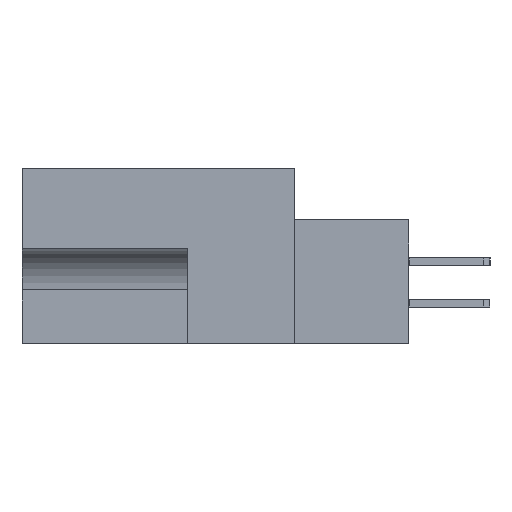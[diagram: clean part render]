
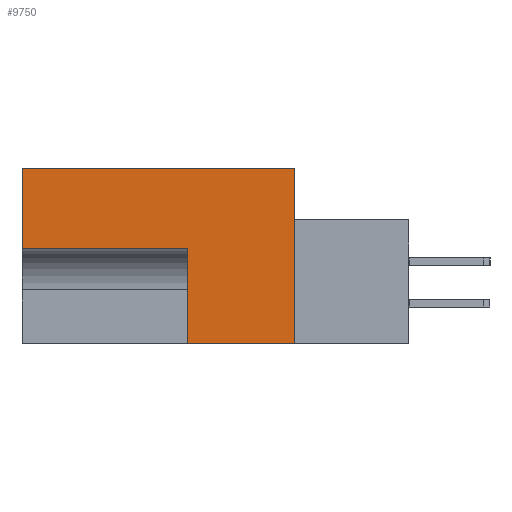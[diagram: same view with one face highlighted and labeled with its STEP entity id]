
A CAD part, left-side view. The second image highlights one B-rep face of the part: STEP entity #9750.
In plain terms, the highlighted planar face has unit normal (-1, 0, 0).
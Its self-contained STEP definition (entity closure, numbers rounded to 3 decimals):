
#291 = LINE ( 'NONE', #34752, #33933 ) ;
#448 = DIRECTION ( 'NONE',  ( 0., -1., 0. ) ) ;
#819 = CARTESIAN_POINT ( 'NONE',  ( 0., 8.255, -6.172 ) ) ;
#1312 = CARTESIAN_POINT ( 'NONE',  ( 0., 20.955, -6.172 ) ) ;
#2213 = EDGE_CURVE ( 'NONE', #24763, #22012, #15601, .T. ) ;
#3023 = PLANE ( 'NONE',  #30456 ) ;
#4687 = LINE ( 'NONE', #26332, #26535 ) ;
#4724 = DIRECTION ( 'NONE',  ( 0., 0., 1. ) ) ;
#9750 = ADVANCED_FACE ( 'NONE', ( #41322 ), #3023, .F. ) ;
#10180 = DIRECTION ( 'NONE',  ( 0., 0., -1. ) ) ;
#11584 = EDGE_CURVE ( 'NONE', #35390, #37635, #27273, .T. ) ;
#12040 = EDGE_CURVE ( 'NONE', #22012, #35390, #291, .T. ) ;
#12641 = VECTOR ( 'NONE', #21623, 1000. ) ;
#12754 = CARTESIAN_POINT ( 'NONE',  ( 0., 0., 0. ) ) ;
#14166 = ORIENTED_EDGE ( 'NONE', *, *, #42905, .F. ) ;
#14206 = ORIENTED_EDGE ( 'NONE', *, *, #12040, .F. ) ;
#15601 = LINE ( 'NONE', #43715, #16158 ) ;
#16158 = VECTOR ( 'NONE', #448, 1000. ) ;
#16974 = EDGE_CURVE ( 'NONE', #21057, #24763, #26714, .T. ) ;
#17038 = ORIENTED_EDGE ( 'NONE', *, *, #2213, .F. ) ;
#18081 = VERTEX_POINT ( 'NONE', #819 ) ;
#19223 = ORIENTED_EDGE ( 'NONE', *, *, #16974, .F. ) ;
#20520 = ORIENTED_EDGE ( 'NONE', *, *, #26386, .F. ) ;
#20882 = CARTESIAN_POINT ( 'NONE',  ( 0., 20.955, -13.487 ) ) ;
#21007 = CARTESIAN_POINT ( 'NONE',  ( 0., 20.955, 0. ) ) ;
#21057 = VERTEX_POINT ( 'NONE', #1312 ) ;
#21623 = DIRECTION ( 'NONE',  ( 0., 1., 0. ) ) ;
#21773 = CARTESIAN_POINT ( 'NONE',  ( 0., -8.814, -13.487 ) ) ;
#22012 = VERTEX_POINT ( 'NONE', #12754 ) ;
#22852 = VECTOR ( 'NONE', #39650, 1000. ) ;
#24763 = VERTEX_POINT ( 'NONE', #21007 ) ;
#25149 = CARTESIAN_POINT ( 'NONE',  ( 0., 8.255, -6.172 ) ) ;
#26309 = CARTESIAN_POINT ( 'NONE',  ( 0., 0., -13.487 ) ) ;
#26332 = CARTESIAN_POINT ( 'NONE',  ( 0., 8.255, -13.487 ) ) ;
#26386 = EDGE_CURVE ( 'NONE', #37635, #18081, #4687, .T. ) ;
#26535 = VECTOR ( 'NONE', #4724, 1000. ) ;
#26714 = LINE ( 'NONE', #20882, #34507 ) ;
#27273 = LINE ( 'NONE', #21773, #12641 ) ;
#28097 = CARTESIAN_POINT ( 'NONE',  ( 0., 0., 0. ) ) ;
#30456 = AXIS2_PLACEMENT_3D ( 'NONE', #28097, #31677, #10180 ) ;
#31677 = DIRECTION ( 'NONE',  ( 1., 0., 0. ) ) ;
#33933 = VECTOR ( 'NONE', #41955, 1000. ) ;
#34507 = VECTOR ( 'NONE', #46083, 1000. ) ;
#34752 = CARTESIAN_POINT ( 'NONE',  ( 0., 0., 0. ) ) ;
#35390 = VERTEX_POINT ( 'NONE', #26309 ) ;
#37139 = ORIENTED_EDGE ( 'NONE', *, *, #11584, .F. ) ;
#37387 = EDGE_LOOP ( 'NONE', ( #37139, #14206, #17038, #19223, #14166, #20520 ) ) ;
#37635 = VERTEX_POINT ( 'NONE', #40234 ) ;
#39650 = DIRECTION ( 'NONE',  ( 0., 1., 0. ) ) ;
#40234 = CARTESIAN_POINT ( 'NONE',  ( 0., 8.255, -13.487 ) ) ;
#41322 = FACE_OUTER_BOUND ( 'NONE', #37387, .T. ) ;
#41955 = DIRECTION ( 'NONE',  ( 0., 0., -1. ) ) ;
#42905 = EDGE_CURVE ( 'NONE', #18081, #21057, #44105, .T. ) ;
#43715 = CARTESIAN_POINT ( 'NONE',  ( 0., 11.506, 0. ) ) ;
#44105 = LINE ( 'NONE', #25149, #22852 ) ;
#46083 = DIRECTION ( 'NONE',  ( 0., 0., 1. ) ) ;
